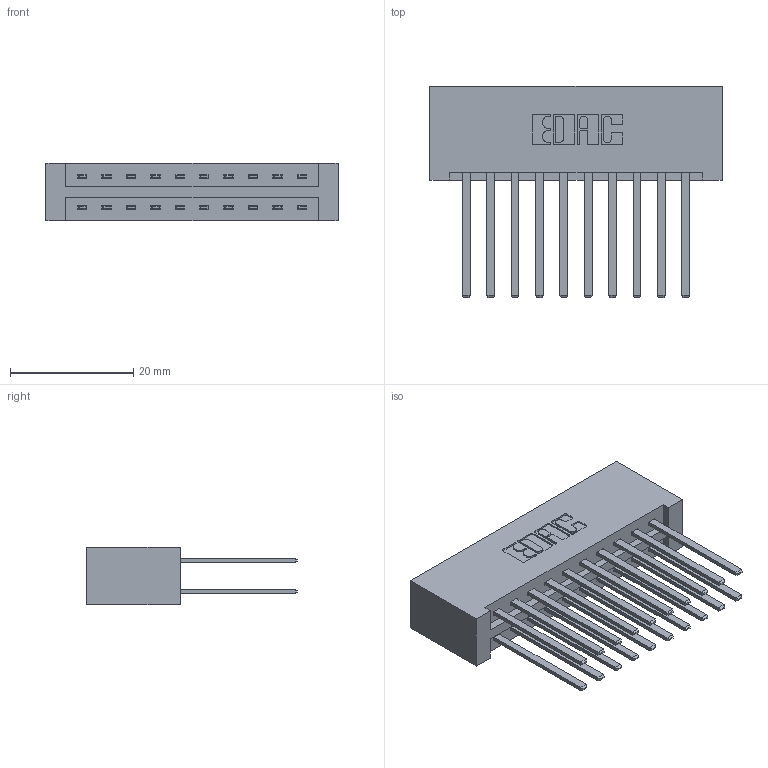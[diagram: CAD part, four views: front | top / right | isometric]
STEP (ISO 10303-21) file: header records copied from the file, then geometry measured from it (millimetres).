
FILE_DESCRIPTION (( 'STEP AP203' ), '1' );
FILE_NAME ('337-020-544-201.STEP', '2018-08-05T09:46:10', ( '' ), ( '' ), 'SwSTEP 2.0', 'SolidWorks 2016', '' );
FILE_SCHEMA (( 'CONFIG_CONTROL_DESIGN' ));
Length unit declared in the file: inch
Products named in the file (3): 337 Part_No Mounting Lugs; 345-292-001_345-293-144; 337-020-544-201
Assembly tree (21 placements, depth 2):
  337-020-544-201
    337 Part_No Mounting Lugs
    345-292-001_345-293-144  x20
Bounding box: 47.5 x 34.3 x 9.4 mm (x, y, z)
Volume: 5620.9 mm3; surface area: 7015.5 mm2
Topology: 21 solids, 21 shells, 1066 faces, 3147 edges, 2070 vertices
Faces by surface type: plane 746, cylinder 320
Entity records: 11431 total; most frequent: CARTESIAN_POINT 1950, ORIENTED_EDGE 1886, DIRECTION 1707, EDGE_CURVE 943, LINE 827, VECTOR 827, VERTEX_POINT 626, AXIS2_PLACEMENT_3D 440
